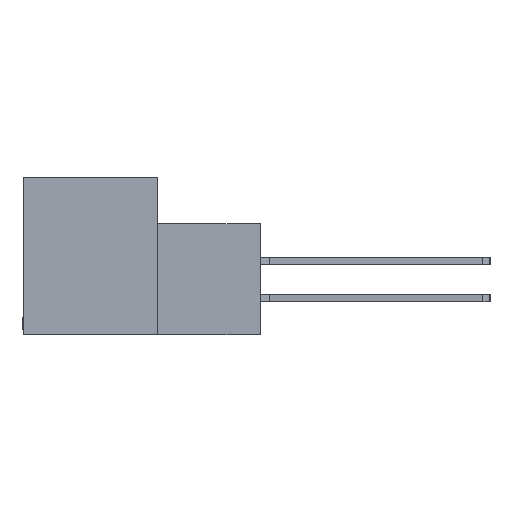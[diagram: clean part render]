
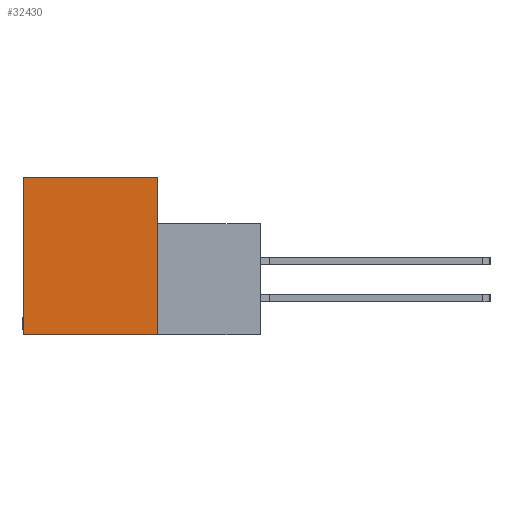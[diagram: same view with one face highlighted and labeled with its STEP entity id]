
A CAD part, left-side view. The second image highlights one B-rep face of the part: STEP entity #32430.
In plain terms, the highlighted planar face has unit normal (-1, 0, 0).
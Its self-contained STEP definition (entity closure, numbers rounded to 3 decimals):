
#368 = DIRECTION ( 'NONE',  ( 0., 0., -1. ) ) ;
#497 = CARTESIAN_POINT ( 'NONE',  ( 0., 11.506, -13.487 ) ) ;
#1339 = AXIS2_PLACEMENT_3D ( 'NONE', #28410, #18242, #368 ) ;
#2494 = CARTESIAN_POINT ( 'NONE',  ( 0., 11.506, 0. ) ) ;
#2496 = CARTESIAN_POINT ( 'NONE',  ( 0., 0., -13.487 ) ) ;
#3117 = FACE_OUTER_BOUND ( 'NONE', #4862, .T. ) ;
#3233 = DIRECTION ( 'NONE',  ( 0., 0., -1. ) ) ;
#3743 = DIRECTION ( 'NONE',  ( 0., -1., 0. ) ) ;
#4862 = EDGE_LOOP ( 'NONE', ( #15737, #14448, #34997, #37054 ) ) ;
#5620 = EDGE_CURVE ( 'NONE', #24972, #40447, #45413, .T. ) ;
#7143 = CARTESIAN_POINT ( 'NONE',  ( 0., 0., 0. ) ) ;
#8192 = EDGE_CURVE ( 'NONE', #40447, #32024, #36922, .T. ) ;
#10530 = CARTESIAN_POINT ( 'NONE',  ( 0., 11.506, 0. ) ) ;
#14448 = ORIENTED_EDGE ( 'NONE', *, *, #5620, .F. ) ;
#15737 = ORIENTED_EDGE ( 'NONE', *, *, #8192, .F. ) ;
#18113 = VECTOR ( 'NONE', #41352, 1000. ) ;
#18242 = DIRECTION ( 'NONE',  ( 1., 0., 0. ) ) ;
#19125 = CARTESIAN_POINT ( 'NONE',  ( 0., -8.814, -13.487 ) ) ;
#21850 = EDGE_CURVE ( 'NONE', #41806, #24972, #39134, .T. ) ;
#24972 = VERTEX_POINT ( 'NONE', #7143 ) ;
#25552 = VECTOR ( 'NONE', #44135, 1000. ) ;
#28410 = CARTESIAN_POINT ( 'NONE',  ( 0., 0., 0. ) ) ;
#29735 = CARTESIAN_POINT ( 'NONE',  ( 0., 11.506, -13.487 ) ) ;
#32024 = VERTEX_POINT ( 'NONE', #497 ) ;
#32430 = ADVANCED_FACE ( 'NONE', ( #3117 ), #35698, .F. ) ;
#33366 = LINE ( 'NONE', #29735, #25552 ) ;
#33817 = VECTOR ( 'NONE', #3233, 1000. ) ;
#34997 = ORIENTED_EDGE ( 'NONE', *, *, #21850, .F. ) ;
#35698 = PLANE ( 'NONE',  #1339 ) ;
#36922 = LINE ( 'NONE', #19125, #18113 ) ;
#36929 = VECTOR ( 'NONE', #3743, 1000. ) ;
#37054 = ORIENTED_EDGE ( 'NONE', *, *, #44579, .F. ) ;
#39134 = LINE ( 'NONE', #10530, #36929 ) ;
#40447 = VERTEX_POINT ( 'NONE', #2496 ) ;
#41352 = DIRECTION ( 'NONE',  ( 0., 1., 0. ) ) ;
#41806 = VERTEX_POINT ( 'NONE', #2494 ) ;
#42269 = CARTESIAN_POINT ( 'NONE',  ( 0., 0., 0. ) ) ;
#44135 = DIRECTION ( 'NONE',  ( 0., 0., 1. ) ) ;
#44579 = EDGE_CURVE ( 'NONE', #32024, #41806, #33366, .T. ) ;
#45413 = LINE ( 'NONE', #42269, #33817 ) ;
